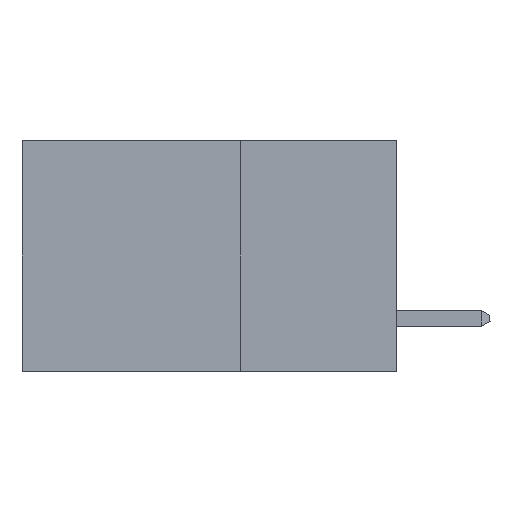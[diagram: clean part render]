
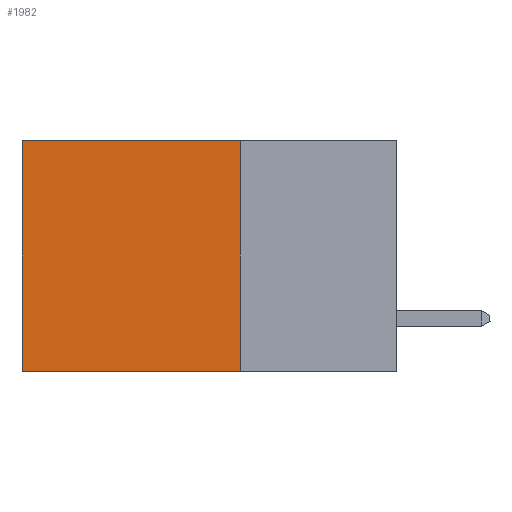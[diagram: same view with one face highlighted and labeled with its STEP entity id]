
A CAD part, left-side view. The second image highlights one B-rep face of the part: STEP entity #1982.
In plain terms, the highlighted planar face has unit normal (-1, 0, 0).
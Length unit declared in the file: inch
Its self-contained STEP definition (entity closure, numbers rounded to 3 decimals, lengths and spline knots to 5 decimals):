
#457 = EDGE_CURVE ( 'NONE', #3812, #9641, #8488, .T. ) ;
#481 = ORIENTED_EDGE ( 'NONE', *, *, #1753, .F. ) ;
#1005 = CARTESIAN_POINT ( 'NONE',  ( 0.298, 0.25, 0. ) ) ;
#1428 = DIRECTION ( 'NONE',  ( 0., 0., -1. ) ) ;
#1646 = PLANE ( 'NONE',  #2255 ) ;
#1753 = EDGE_CURVE ( 'NONE', #9518, #6769, #9063, .T. ) ;
#1982 = ADVANCED_FACE ( 'NONE', ( #10736 ), #1646, .F. ) ;
#2227 = ORIENTED_EDGE ( 'NONE', *, *, #2366, .T. ) ;
#2255 = AXIS2_PLACEMENT_3D ( 'NONE', #4024, #10922, #7743 ) ;
#2366 = EDGE_CURVE ( 'NONE', #9518, #3812, #5133, .T. ) ;
#3389 = CARTESIAN_POINT ( 'NONE',  ( 0.298, 0.25, 0. ) ) ;
#3569 = VECTOR ( 'NONE', #11358, 39.37008 ) ;
#3812 = VERTEX_POINT ( 'NONE', #10661 ) ;
#4024 = CARTESIAN_POINT ( 'NONE',  ( 0.298, 0.25, 0. ) ) ;
#4098 = CARTESIAN_POINT ( 'NONE',  ( 0.298, 0.25, -0.37 ) ) ;
#4283 = ORIENTED_EDGE ( 'NONE', *, *, #11425, .F. ) ;
#4410 = VECTOR ( 'NONE', #1428, 39.37008 ) ;
#4669 = CARTESIAN_POINT ( 'NONE',  ( 0.298, 0.25, 0. ) ) ;
#5067 = CARTESIAN_POINT ( 'NONE',  ( 0.298, 0.6, 0. ) ) ;
#5133 = LINE ( 'NONE', #3389, #7594 ) ;
#5219 = CARTESIAN_POINT ( 'NONE',  ( 0.298, 0.25, -0.37 ) ) ;
#5742 = CARTESIAN_POINT ( 'NONE',  ( 0.298, 0.6, -0.37 ) ) ;
#6266 = EDGE_LOOP ( 'NONE', ( #9476, #4283, #481, #2227 ) ) ;
#6769 = VERTEX_POINT ( 'NONE', #5219 ) ;
#7594 = VECTOR ( 'NONE', #11195, 39.37008 ) ;
#7743 = DIRECTION ( 'NONE',  ( 0., 0., -1. ) ) ;
#8271 = VECTOR ( 'NONE', #11412, 39.37008 ) ;
#8488 = LINE ( 'NONE', #5067, #3569 ) ;
#8568 = LINE ( 'NONE', #4098, #8271 ) ;
#9063 = LINE ( 'NONE', #1005, #4410 ) ;
#9476 = ORIENTED_EDGE ( 'NONE', *, *, #457, .T. ) ;
#9518 = VERTEX_POINT ( 'NONE', #4669 ) ;
#9641 = VERTEX_POINT ( 'NONE', #5742 ) ;
#10661 = CARTESIAN_POINT ( 'NONE',  ( 0.298, 0.6, 0. ) ) ;
#10736 = FACE_OUTER_BOUND ( 'NONE', #6266, .T. ) ;
#10922 = DIRECTION ( 'NONE',  ( 1., 0., 0. ) ) ;
#11195 = DIRECTION ( 'NONE',  ( 0., 1., 0. ) ) ;
#11358 = DIRECTION ( 'NONE',  ( 0., 0., -1. ) ) ;
#11412 = DIRECTION ( 'NONE',  ( 0., 1., 0. ) ) ;
#11425 = EDGE_CURVE ( 'NONE', #6769, #9641, #8568, .T. ) ;
